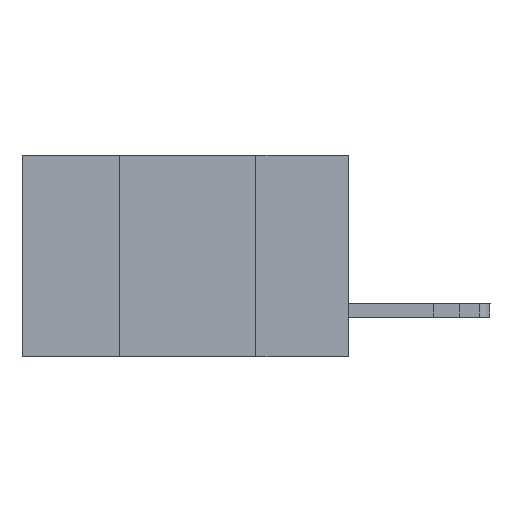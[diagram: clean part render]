
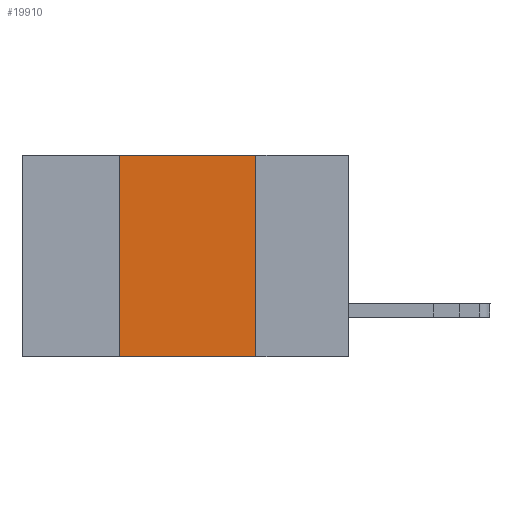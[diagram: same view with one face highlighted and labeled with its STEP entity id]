
A CAD part, left-side view. The second image highlights one B-rep face of the part: STEP entity #19910.
In plain terms, the highlighted planar face has unit normal (-1, 0, 0).
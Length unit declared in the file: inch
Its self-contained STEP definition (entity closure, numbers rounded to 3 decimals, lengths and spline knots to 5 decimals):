
#495 = FACE_OUTER_BOUND ( 'NONE', #15947, .T. ) ;
#2781 = CARTESIAN_POINT ( 'NONE',  ( 0., 0.42, 0. ) ) ;
#3681 = CARTESIAN_POINT ( 'NONE',  ( 0., 0.6, 0. ) ) ;
#3865 = LINE ( 'NONE', #10017, #18158 ) ;
#4454 = VERTEX_POINT ( 'NONE', #5160 ) ;
#4497 = LINE ( 'NONE', #10659, #13942 ) ;
#4648 = DIRECTION ( 'NONE',  ( 0., 0., 1. ) ) ;
#5160 = CARTESIAN_POINT ( 'NONE',  ( 0., 0.17, 0. ) ) ;
#5629 = VERTEX_POINT ( 'NONE', #2781 ) ;
#5854 = LINE ( 'NONE', #13726, #7948 ) ;
#7612 = CARTESIAN_POINT ( 'NONE',  ( 0., 0.42, -0.37 ) ) ;
#7730 = DIRECTION ( 'NONE',  ( 0., 0., -1. ) ) ;
#7796 = VERTEX_POINT ( 'NONE', #10510 ) ;
#7948 = VECTOR ( 'NONE', #9281, 39.37008 ) ;
#8041 = ORIENTED_EDGE ( 'NONE', *, *, #13412, .F. ) ;
#8446 = EDGE_CURVE ( 'NONE', #5629, #4454, #5854, .T. ) ;
#9164 = DIRECTION ( 'NONE',  ( 0., -1., 0. ) ) ;
#9259 = CARTESIAN_POINT ( 'NONE',  ( 0., 0.17, -0.37 ) ) ;
#9281 = DIRECTION ( 'NONE',  ( 0., -1., 0. ) ) ;
#9906 = VERTEX_POINT ( 'NONE', #7612 ) ;
#10017 = CARTESIAN_POINT ( 'NONE',  ( 0., 0.42, -0.37 ) ) ;
#10287 = VECTOR ( 'NONE', #7730, 39.37008 ) ;
#10510 = CARTESIAN_POINT ( 'NONE',  ( 0., 0.17, -0.37 ) ) ;
#10659 = CARTESIAN_POINT ( 'NONE',  ( 0., 0.6, -0.37 ) ) ;
#11511 = ORIENTED_EDGE ( 'NONE', *, *, #17716, .F. ) ;
#12284 = ORIENTED_EDGE ( 'NONE', *, *, #8446, .F. ) ;
#13412 = EDGE_CURVE ( 'NONE', #4454, #7796, #16923, .T. ) ;
#13663 = AXIS2_PLACEMENT_3D ( 'NONE', #3681, #16283, #14747 ) ;
#13726 = CARTESIAN_POINT ( 'NONE',  ( 0., 0.6, 0. ) ) ;
#13942 = VECTOR ( 'NONE', #9164, 39.37008 ) ;
#14747 = DIRECTION ( 'NONE',  ( 0., 0., -1. ) ) ;
#15947 = EDGE_LOOP ( 'NONE', ( #8041, #12284, #11511, #18175 ) ) ;
#16283 = DIRECTION ( 'NONE',  ( 1., 0., 0. ) ) ;
#16923 = LINE ( 'NONE', #9259, #10287 ) ;
#17517 = EDGE_CURVE ( 'NONE', #9906, #7796, #4497, .T. ) ;
#17716 = EDGE_CURVE ( 'NONE', #9906, #5629, #3865, .T. ) ;
#17801 = PLANE ( 'NONE',  #13663 ) ;
#18158 = VECTOR ( 'NONE', #4648, 39.37008 ) ;
#18175 = ORIENTED_EDGE ( 'NONE', *, *, #17517, .T. ) ;
#19910 = ADVANCED_FACE ( 'NONE', ( #495 ), #17801, .F. ) ;
